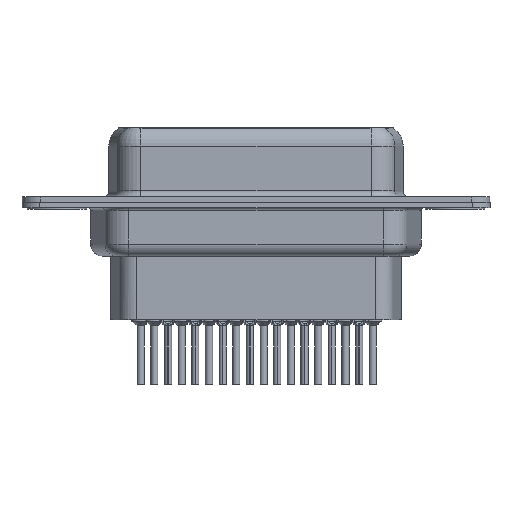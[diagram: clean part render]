
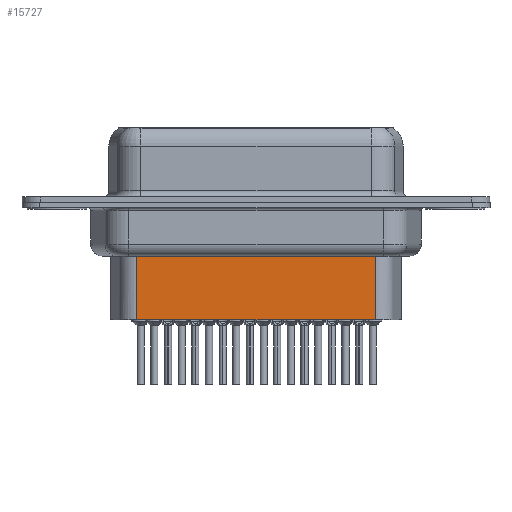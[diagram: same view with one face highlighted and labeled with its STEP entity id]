
A CAD part, front view. The second image highlights one B-rep face of the part: STEP entity #15727.
In plain terms, the highlighted planar face has unit normal (0, -1, 0).
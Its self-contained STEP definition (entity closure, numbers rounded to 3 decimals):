
#722 = EDGE_CURVE ( 'NONE', #19350, #28176, #24205, .T. ) ;
#2106 = DIRECTION ( 'NONE',  ( 0., 0., -1. ) ) ;
#2151 = EDGE_CURVE ( 'NONE', #21677, #27128, #7404, .T. ) ;
#2802 = DIRECTION ( 'NONE',  ( -1., 0., 0. ) ) ;
#2808 = CARTESIAN_POINT ( 'NONE',  ( 6.691, -3.5, -3.1 ) ) ;
#4226 = VECTOR ( 'NONE', #2106, 1000. ) ;
#5908 = VECTOR ( 'NONE', #2802, 1000. ) ;
#7404 = LINE ( 'NONE', #28347, #4226 ) ;
#7934 = CARTESIAN_POINT ( 'NONE',  ( 26.629, -3.5, -9.85 ) ) ;
#8833 = VECTOR ( 'NONE', #9219, 1000. ) ;
#9219 = DIRECTION ( 'NONE',  ( -1., 0., 0. ) ) ;
#10263 = LINE ( 'NONE', #19197, #5908 ) ;
#11367 = AXIS2_PLACEMENT_3D ( 'NONE', #28463, #14230, #23776 ) ;
#13656 = CARTESIAN_POINT ( 'NONE',  ( 26.629, -3.5, -4.097 ) ) ;
#13929 = CARTESIAN_POINT ( 'NONE',  ( 6.691, -3.5, -9.85 ) ) ;
#14230 = DIRECTION ( 'NONE',  ( 0., -1., 0. ) ) ;
#15727 = ADVANCED_FACE ( 'NONE', ( #30817 ), #18924, .T. ) ;
#17400 = EDGE_CURVE ( 'NONE', #21677, #19350, #10263, .T. ) ;
#17902 = ORIENTED_EDGE ( 'NONE', *, *, #722, .T. ) ;
#18056 = EDGE_LOOP ( 'NONE', ( #18134, #23990, #17902, #20821 ) ) ;
#18134 = ORIENTED_EDGE ( 'NONE', *, *, #2151, .F. ) ;
#18924 = PLANE ( 'NONE',  #11367 ) ;
#19045 = DIRECTION ( 'NONE',  ( 0., 0., -1. ) ) ;
#19197 = CARTESIAN_POINT ( 'NONE',  ( 6.444, -3.5, -4.097 ) ) ;
#19350 = VERTEX_POINT ( 'NONE', #25521 ) ;
#20821 = ORIENTED_EDGE ( 'NONE', *, *, #30874, .F. ) ;
#21677 = VERTEX_POINT ( 'NONE', #13656 ) ;
#23776 = DIRECTION ( 'NONE',  ( 1., 0., 0. ) ) ;
#23990 = ORIENTED_EDGE ( 'NONE', *, *, #17400, .T. ) ;
#24205 = LINE ( 'NONE', #2808, #26574 ) ;
#25521 = CARTESIAN_POINT ( 'NONE',  ( 6.691, -3.5, -4.097 ) ) ;
#26574 = VECTOR ( 'NONE', #19045, 1000. ) ;
#27128 = VERTEX_POINT ( 'NONE', #7934 ) ;
#27991 = LINE ( 'NONE', #28442, #8833 ) ;
#28176 = VERTEX_POINT ( 'NONE', #13929 ) ;
#28347 = CARTESIAN_POINT ( 'NONE',  ( 26.629, -3.5, -3.1 ) ) ;
#28442 = CARTESIAN_POINT ( 'NONE',  ( 6.691, -3.5, -9.85 ) ) ;
#28463 = CARTESIAN_POINT ( 'NONE',  ( 6.691, -3.5, -3.1 ) ) ;
#30817 = FACE_OUTER_BOUND ( 'NONE', #18056, .T. ) ;
#30874 = EDGE_CURVE ( 'NONE', #27128, #28176, #27991, .T. ) ;
